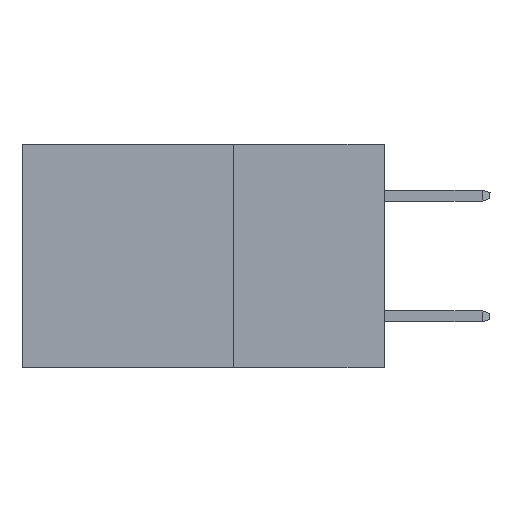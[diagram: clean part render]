
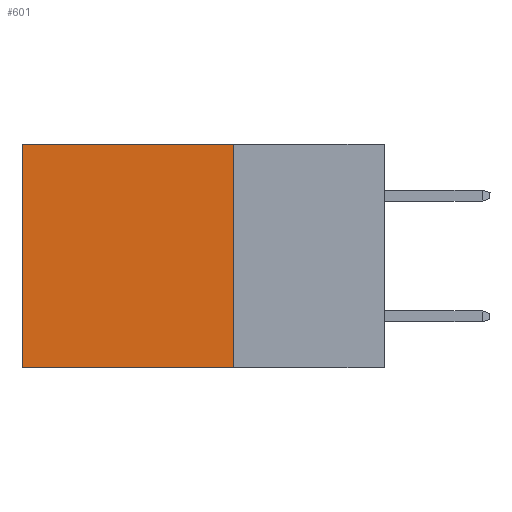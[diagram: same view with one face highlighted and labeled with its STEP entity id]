
A CAD part, left-side view. The second image highlights one B-rep face of the part: STEP entity #601.
In plain terms, the highlighted planar face has unit normal (-1, 0, 0).
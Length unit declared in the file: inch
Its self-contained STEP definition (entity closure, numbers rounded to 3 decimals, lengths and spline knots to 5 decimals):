
#135 = DIRECTION ( 'NONE',  ( 1., 0., 0. ) ) ;
#601 = ADVANCED_FACE ( 'NONE', ( #6004 ), #7462, .F. ) ;
#644 = VERTEX_POINT ( 'NONE', #9141 ) ;
#1055 = DIRECTION ( 'NONE',  ( 0., 1., 0. ) ) ;
#2882 = CARTESIAN_POINT ( 'NONE',  ( 0.298, 0.6, -0.37 ) ) ;
#3087 = VERTEX_POINT ( 'NONE', #3967 ) ;
#3160 = LINE ( 'NONE', #6955, #5244 ) ;
#3209 = AXIS2_PLACEMENT_3D ( 'NONE', #4119, #135, #3320 ) ;
#3320 = DIRECTION ( 'NONE',  ( 0., 0., -1. ) ) ;
#3417 = LINE ( 'NONE', #5970, #9791 ) ;
#3719 = VERTEX_POINT ( 'NONE', #8004 ) ;
#3731 = EDGE_LOOP ( 'NONE', ( #7745, #9909, #5522, #9400 ) ) ;
#3777 = EDGE_CURVE ( 'NONE', #3087, #10535, #8558, .T. ) ;
#3967 = CARTESIAN_POINT ( 'NONE',  ( 0.298, 0.6, 0. ) ) ;
#4119 = CARTESIAN_POINT ( 'NONE',  ( 0.298, 0.25, 0. ) ) ;
#4268 = EDGE_CURVE ( 'NONE', #644, #3087, #3160, .T. ) ;
#5174 = LINE ( 'NONE', #10324, #7472 ) ;
#5244 = VECTOR ( 'NONE', #9430, 39.37008 ) ;
#5522 = ORIENTED_EDGE ( 'NONE', *, *, #6801, .F. ) ;
#5970 = CARTESIAN_POINT ( 'NONE',  ( 0.298, 0.25, -0.37 ) ) ;
#6004 = FACE_OUTER_BOUND ( 'NONE', #3731, .T. ) ;
#6538 = VECTOR ( 'NONE', #8719, 39.37008 ) ;
#6801 = EDGE_CURVE ( 'NONE', #644, #3719, #5174, .T. ) ;
#6955 = CARTESIAN_POINT ( 'NONE',  ( 0.298, 0.25, 0. ) ) ;
#7462 = PLANE ( 'NONE',  #3209 ) ;
#7472 = VECTOR ( 'NONE', #7949, 39.37008 ) ;
#7745 = ORIENTED_EDGE ( 'NONE', *, *, #3777, .T. ) ;
#7949 = DIRECTION ( 'NONE',  ( 0., 0., -1. ) ) ;
#8004 = CARTESIAN_POINT ( 'NONE',  ( 0.298, 0.25, -0.37 ) ) ;
#8558 = LINE ( 'NONE', #9559, #6538 ) ;
#8719 = DIRECTION ( 'NONE',  ( 0., 0., -1. ) ) ;
#8957 = EDGE_CURVE ( 'NONE', #3719, #10535, #3417, .T. ) ;
#9141 = CARTESIAN_POINT ( 'NONE',  ( 0.298, 0.25, 0. ) ) ;
#9400 = ORIENTED_EDGE ( 'NONE', *, *, #4268, .T. ) ;
#9430 = DIRECTION ( 'NONE',  ( 0., 1., 0. ) ) ;
#9559 = CARTESIAN_POINT ( 'NONE',  ( 0.298, 0.6, 0. ) ) ;
#9791 = VECTOR ( 'NONE', #1055, 39.37008 ) ;
#9909 = ORIENTED_EDGE ( 'NONE', *, *, #8957, .F. ) ;
#10324 = CARTESIAN_POINT ( 'NONE',  ( 0.298, 0.25, 0. ) ) ;
#10535 = VERTEX_POINT ( 'NONE', #2882 ) ;
